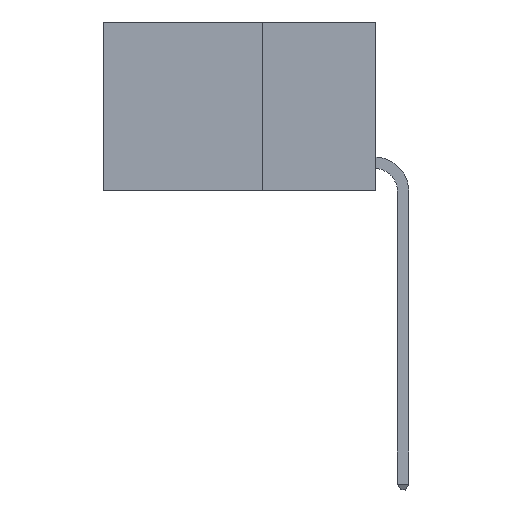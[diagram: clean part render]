
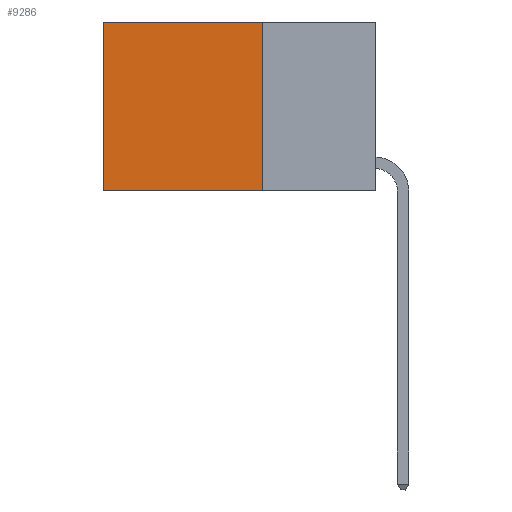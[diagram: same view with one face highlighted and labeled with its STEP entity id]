
A CAD part, left-side view. The second image highlights one B-rep face of the part: STEP entity #9286.
In plain terms, the highlighted planar face has unit normal (-1, 0, 0).
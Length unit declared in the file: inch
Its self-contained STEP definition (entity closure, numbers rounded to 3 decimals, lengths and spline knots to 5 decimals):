
#510 = ORIENTED_EDGE ( 'NONE', *, *, #5548, .F. ) ;
#991 = DIRECTION ( 'NONE',  ( 0., 0., -1. ) ) ;
#1349 = VERTEX_POINT ( 'NONE', #6036 ) ;
#1372 = EDGE_LOOP ( 'NONE', ( #9925, #510, #11093, #2913 ) ) ;
#1410 = LINE ( 'NONE', #15661, #10746 ) ;
#1498 = EDGE_CURVE ( 'NONE', #4001, #1349, #1549, .T. ) ;
#1549 = LINE ( 'NONE', #1793, #4029 ) ;
#1705 = DIRECTION ( 'NONE',  ( 0., 1., 0. ) ) ;
#1793 = CARTESIAN_POINT ( 'NONE',  ( 0.2625, 0.25, 0. ) ) ;
#1968 = VECTOR ( 'NONE', #8530, 39.37008 ) ;
#2352 = LINE ( 'NONE', #15640, #1968 ) ;
#2587 = CARTESIAN_POINT ( 'NONE',  ( 0.2625, 0.25, 0. ) ) ;
#2913 = ORIENTED_EDGE ( 'NONE', *, *, #1498, .T. ) ;
#4001 = VERTEX_POINT ( 'NONE', #13874 ) ;
#4029 = VECTOR ( 'NONE', #1705, 39.37008 ) ;
#4463 = VERTEX_POINT ( 'NONE', #13512 ) ;
#4569 = AXIS2_PLACEMENT_3D ( 'NONE', #15442, #8327, #991 ) ;
#5548 = EDGE_CURVE ( 'NONE', #10747, #4463, #1410, .T. ) ;
#6036 = CARTESIAN_POINT ( 'NONE',  ( 0.2625, 0.6, 0. ) ) ;
#6177 = EDGE_CURVE ( 'NONE', #1349, #4463, #2352, .T. ) ;
#7095 = PLANE ( 'NONE',  #4569 ) ;
#7265 = FACE_OUTER_BOUND ( 'NONE', #1372, .T. ) ;
#8327 = DIRECTION ( 'NONE',  ( 1., 0., 0. ) ) ;
#8530 = DIRECTION ( 'NONE',  ( 0., 0., -1. ) ) ;
#8542 = LINE ( 'NONE', #2587, #11360 ) ;
#9286 = ADVANCED_FACE ( 'NONE', ( #7265 ), #7095, .F. ) ;
#9760 = DIRECTION ( 'NONE',  ( 0., 1., 0. ) ) ;
#9886 = DIRECTION ( 'NONE',  ( 0., 0., -1. ) ) ;
#9925 = ORIENTED_EDGE ( 'NONE', *, *, #6177, .T. ) ;
#10746 = VECTOR ( 'NONE', #9760, 39.37008 ) ;
#10747 = VERTEX_POINT ( 'NONE', #13832 ) ;
#11093 = ORIENTED_EDGE ( 'NONE', *, *, #11840, .F. ) ;
#11360 = VECTOR ( 'NONE', #9886, 39.37008 ) ;
#11840 = EDGE_CURVE ( 'NONE', #4001, #10747, #8542, .T. ) ;
#13512 = CARTESIAN_POINT ( 'NONE',  ( 0.2625, 0.6, -0.37 ) ) ;
#13832 = CARTESIAN_POINT ( 'NONE',  ( 0.2625, 0.25, -0.37 ) ) ;
#13874 = CARTESIAN_POINT ( 'NONE',  ( 0.2625, 0.25, 0. ) ) ;
#15442 = CARTESIAN_POINT ( 'NONE',  ( 0.2625, 0.25, 0. ) ) ;
#15640 = CARTESIAN_POINT ( 'NONE',  ( 0.2625, 0.6, 0. ) ) ;
#15661 = CARTESIAN_POINT ( 'NONE',  ( 0.2625, 0.25, -0.37 ) ) ;
